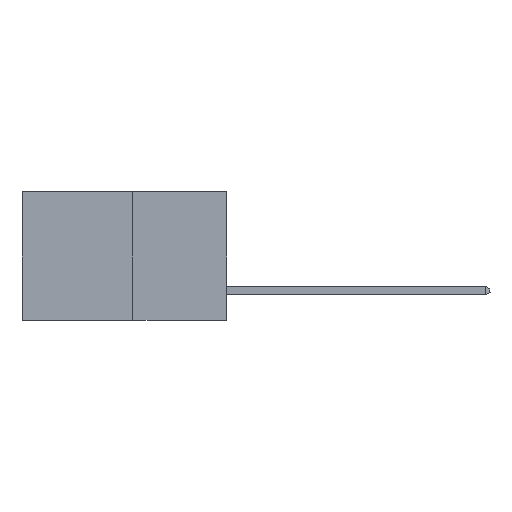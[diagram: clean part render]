
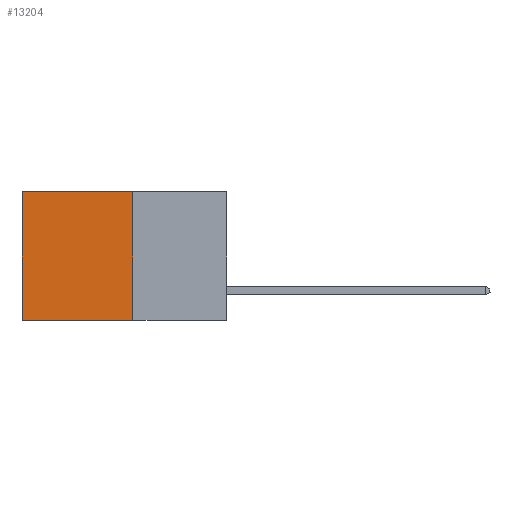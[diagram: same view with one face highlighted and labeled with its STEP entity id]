
A CAD part, left-side view. The second image highlights one B-rep face of the part: STEP entity #13204.
In plain terms, the highlighted planar face has unit normal (-1, 0, 0).
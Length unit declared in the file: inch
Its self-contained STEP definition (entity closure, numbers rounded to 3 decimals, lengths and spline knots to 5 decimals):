
#404 = EDGE_CURVE ( 'NONE', #4973, #5636, #16396, .T. ) ;
#763 = VECTOR ( 'NONE', #5706, 39.37008 ) ;
#1016 = AXIS2_PLACEMENT_3D ( 'NONE', #17952, #8618, #19438 ) ;
#1251 = LINE ( 'NONE', #13719, #763 ) ;
#2790 = ORIENTED_EDGE ( 'NONE', *, *, #18906, .T. ) ;
#3879 = VERTEX_POINT ( 'NONE', #8917 ) ;
#4160 = EDGE_LOOP ( 'NONE', ( #7901, #5088, #4678, #2790 ) ) ;
#4170 = CARTESIAN_POINT ( 'NONE',  ( 0.277, 0.59, -0.37 ) ) ;
#4495 = DIRECTION ( 'NONE',  ( 0., 0., -1. ) ) ;
#4678 = ORIENTED_EDGE ( 'NONE', *, *, #4977, .F. ) ;
#4973 = VERTEX_POINT ( 'NONE', #9838 ) ;
#4977 = EDGE_CURVE ( 'NONE', #13624, #3879, #14623, .T. ) ;
#5088 = ORIENTED_EDGE ( 'NONE', *, *, #7488, .F. ) ;
#5636 = VERTEX_POINT ( 'NONE', #17731 ) ;
#5706 = DIRECTION ( 'NONE',  ( 0., 1., 0. ) ) ;
#7488 = EDGE_CURVE ( 'NONE', #3879, #5636, #16379, .T. ) ;
#7901 = ORIENTED_EDGE ( 'NONE', *, *, #404, .T. ) ;
#8040 = VECTOR ( 'NONE', #4495, 39.37008 ) ;
#8618 = DIRECTION ( 'NONE',  ( 1., 0., 0. ) ) ;
#8917 = CARTESIAN_POINT ( 'NONE',  ( 0.277, 0.27, -0.37 ) ) ;
#9838 = CARTESIAN_POINT ( 'NONE',  ( 0.277, 0.59, 0. ) ) ;
#11454 = FACE_OUTER_BOUND ( 'NONE', #4160, .T. ) ;
#13204 = ADVANCED_FACE ( 'NONE', ( #11454 ), #13387, .F. ) ;
#13387 = PLANE ( 'NONE',  #1016 ) ;
#13624 = VERTEX_POINT ( 'NONE', #15928 ) ;
#13719 = CARTESIAN_POINT ( 'NONE',  ( 0.277, 0.27, 0. ) ) ;
#14623 = LINE ( 'NONE', #19302, #17691 ) ;
#15417 = DIRECTION ( 'NONE',  ( 0., 1., 0. ) ) ;
#15496 = CARTESIAN_POINT ( 'NONE',  ( 0.277, 0.27, -0.37 ) ) ;
#15928 = CARTESIAN_POINT ( 'NONE',  ( 0.277, 0.27, 0. ) ) ;
#15931 = VECTOR ( 'NONE', #15417, 39.37008 ) ;
#16379 = LINE ( 'NONE', #15496, #15931 ) ;
#16396 = LINE ( 'NONE', #4170, #8040 ) ;
#16763 = DIRECTION ( 'NONE',  ( 0., 0., -1. ) ) ;
#17691 = VECTOR ( 'NONE', #16763, 39.37008 ) ;
#17731 = CARTESIAN_POINT ( 'NONE',  ( 0.277, 0.59, -0.37 ) ) ;
#17952 = CARTESIAN_POINT ( 'NONE',  ( 0.277, 0.27, -0.37 ) ) ;
#18906 = EDGE_CURVE ( 'NONE', #13624, #4973, #1251, .T. ) ;
#19302 = CARTESIAN_POINT ( 'NONE',  ( 0.277, 0.27, -0.37 ) ) ;
#19438 = DIRECTION ( 'NONE',  ( 0., 0., -1. ) ) ;
